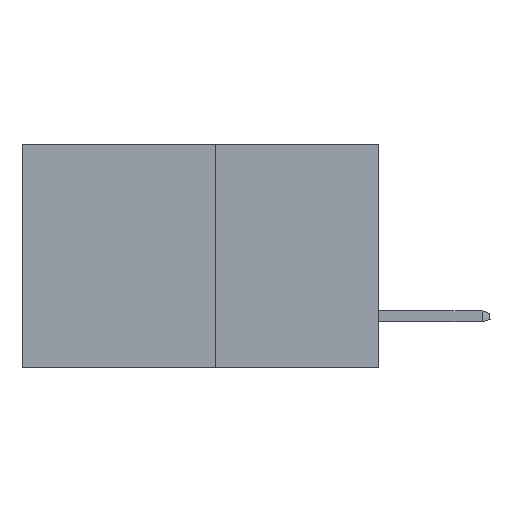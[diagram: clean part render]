
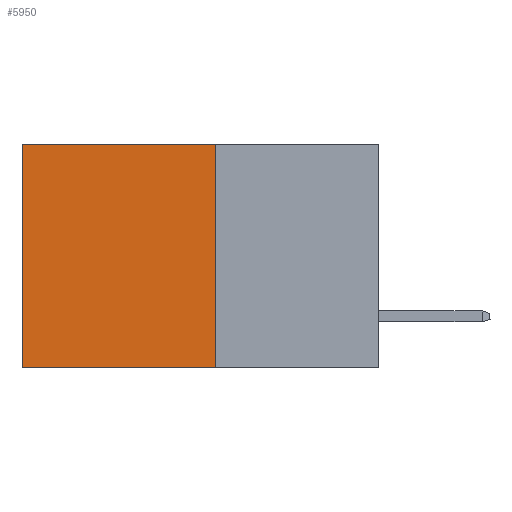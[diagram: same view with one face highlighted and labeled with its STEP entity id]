
A CAD part, left-side view. The second image highlights one B-rep face of the part: STEP entity #5950.
In plain terms, the highlighted planar face has unit normal (-1, 0, 0).
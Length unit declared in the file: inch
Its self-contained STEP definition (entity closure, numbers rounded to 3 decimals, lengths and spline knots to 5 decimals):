
#1193 = CARTESIAN_POINT ( 'NONE',  ( 0.277, 0.27, 0. ) ) ;
#1618 = CARTESIAN_POINT ( 'NONE',  ( 0.277, 0.59, 0. ) ) ;
#1740 = PLANE ( 'NONE',  #16624 ) ;
#2748 = CARTESIAN_POINT ( 'NONE',  ( 0.277, 0.27, 0. ) ) ;
#2972 = VECTOR ( 'NONE', #14229, 39.37008 ) ;
#4500 = CARTESIAN_POINT ( 'NONE',  ( 0.277, 0.59, -0.37 ) ) ;
#4513 = EDGE_CURVE ( 'NONE', #7383, #14068, #6622, .T. ) ;
#4517 = DIRECTION ( 'NONE',  ( 0., 0., -1. ) ) ;
#4671 = LINE ( 'NONE', #1193, #7889 ) ;
#5730 = FACE_OUTER_BOUND ( 'NONE', #14062, .T. ) ;
#5817 = DIRECTION ( 'NONE',  ( 0., 0., -1. ) ) ;
#5950 = ADVANCED_FACE ( 'NONE', ( #5730 ), #1740, .F. ) ;
#6537 = ORIENTED_EDGE ( 'NONE', *, *, #4513, .F. ) ;
#6622 = LINE ( 'NONE', #14971, #2972 ) ;
#7087 = VECTOR ( 'NONE', #11552, 39.37008 ) ;
#7383 = VERTEX_POINT ( 'NONE', #7396 ) ;
#7396 = CARTESIAN_POINT ( 'NONE',  ( 0.277, 0.27, -0.37 ) ) ;
#7527 = LINE ( 'NONE', #10184, #7087 ) ;
#7850 = VERTEX_POINT ( 'NONE', #1618 ) ;
#7889 = VECTOR ( 'NONE', #14771, 39.37008 ) ;
#8771 = ORIENTED_EDGE ( 'NONE', *, *, #12830, .T. ) ;
#10184 = CARTESIAN_POINT ( 'NONE',  ( 0.277, 0.27, -0.37 ) ) ;
#10843 = VERTEX_POINT ( 'NONE', #2748 ) ;
#10873 = VECTOR ( 'NONE', #5817, 39.37008 ) ;
#11064 = EDGE_CURVE ( 'NONE', #10843, #7383, #7527, .T. ) ;
#11324 = CARTESIAN_POINT ( 'NONE',  ( 0.277, 0.27, -0.37 ) ) ;
#11350 = CARTESIAN_POINT ( 'NONE',  ( 0.277, 0.59, -0.37 ) ) ;
#11552 = DIRECTION ( 'NONE',  ( 0., 0., -1. ) ) ;
#12677 = DIRECTION ( 'NONE',  ( 1., 0., 0. ) ) ;
#12830 = EDGE_CURVE ( 'NONE', #7850, #14068, #17433, .T. ) ;
#13848 = EDGE_CURVE ( 'NONE', #10843, #7850, #4671, .T. ) ;
#14062 = EDGE_LOOP ( 'NONE', ( #8771, #6537, #14857, #16388 ) ) ;
#14068 = VERTEX_POINT ( 'NONE', #4500 ) ;
#14229 = DIRECTION ( 'NONE',  ( 0., 1., 0. ) ) ;
#14771 = DIRECTION ( 'NONE',  ( 0., 1., 0. ) ) ;
#14857 = ORIENTED_EDGE ( 'NONE', *, *, #11064, .F. ) ;
#14971 = CARTESIAN_POINT ( 'NONE',  ( 0.277, 0.27, -0.37 ) ) ;
#16388 = ORIENTED_EDGE ( 'NONE', *, *, #13848, .T. ) ;
#16624 = AXIS2_PLACEMENT_3D ( 'NONE', #11324, #12677, #4517 ) ;
#17433 = LINE ( 'NONE', #11350, #10873 ) ;
